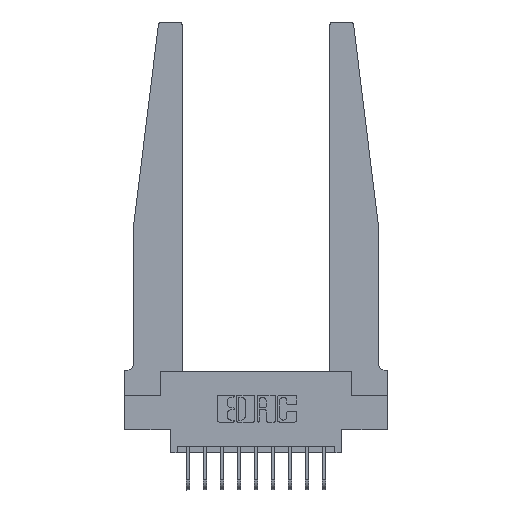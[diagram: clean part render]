
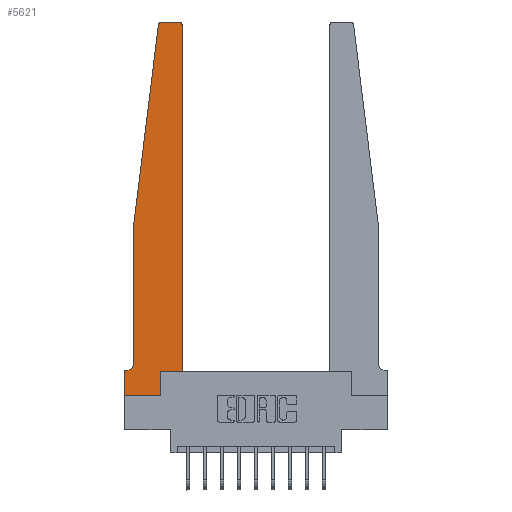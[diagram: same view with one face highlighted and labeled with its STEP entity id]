
A CAD part, top view. The second image highlights one B-rep face of the part: STEP entity #5621.
In plain terms, the highlighted planar face has unit normal (0, 0, 1).
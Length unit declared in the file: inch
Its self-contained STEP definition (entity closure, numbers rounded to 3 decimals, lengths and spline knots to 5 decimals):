
#39 = CARTESIAN_POINT ( 'NONE',  ( 0.2605, 0.18, 0.37 ) ) ;
#132 = CARTESIAN_POINT ( 'NONE',  ( 0.065, 1.25, 0.37 ) ) ;
#312 = EDGE_CURVE ( 'NONE', #11088, #11371, #10918, .T. ) ;
#405 = LINE ( 'NONE', #2624, #12284 ) ;
#443 = DIRECTION ( 'NONE',  ( 0., 0., -1. ) ) ;
#481 = CARTESIAN_POINT ( 'NONE',  ( 0.27653, 2.75, 0.37 ) ) ;
#971 = VERTEX_POINT ( 'NONE', #132 ) ;
#1061 = CARTESIAN_POINT ( 'NONE',  ( 0.2605, 0., 0.37 ) ) ;
#1147 = VECTOR ( 'NONE', #1326, 39.37008 ) ;
#1326 = DIRECTION ( 'NONE',  ( 0., -1., 0. ) ) ;
#1455 = VERTEX_POINT ( 'NONE', #39 ) ;
#1608 = CARTESIAN_POINT ( 'NONE',  ( 0., 0., 0.37 ) ) ;
#2047 = CARTESIAN_POINT ( 'NONE',  ( 0.24675, 2.72367, 0.37 ) ) ;
#2425 = CARTESIAN_POINT ( 'NONE',  ( 0., 0.1875, 0.37 ) ) ;
#2616 = AXIS2_PLACEMENT_3D ( 'NONE', #9842, #3272, #5939 ) ;
#2624 = CARTESIAN_POINT ( 'NONE',  ( 0.25, 2.75, 0.37 ) ) ;
#2648 = CARTESIAN_POINT ( 'NONE',  ( 0.065, 1.25, 0.37 ) ) ;
#2715 = CARTESIAN_POINT ( 'NONE',  ( 0., 0., 0.37 ) ) ;
#2930 = DIRECTION ( 'NONE',  ( 0., 1., 0. ) ) ;
#2935 = CARTESIAN_POINT ( 'NONE',  ( 0.425, 0.18, 0.37 ) ) ;
#3244 = DIRECTION ( 'NONE',  ( -1., 0., 0. ) ) ;
#3258 = ORIENTED_EDGE ( 'NONE', *, *, #13320, .T. ) ;
#3272 = DIRECTION ( 'NONE',  ( 0., 0., 1. ) ) ;
#3311 = EDGE_CURVE ( 'NONE', #971, #10964, #10411, .T. ) ;
#3678 = LINE ( 'NONE', #1608, #16858 ) ;
#4078 = VECTOR ( 'NONE', #11963, 39.37008 ) ;
#4135 = DIRECTION ( 'NONE',  ( 0., -1., 0. ) ) ;
#4272 = DIRECTION ( 'NONE',  ( 0., 1., 0. ) ) ;
#4403 = VERTEX_POINT ( 'NONE', #2715 ) ;
#4493 = ORIENTED_EDGE ( 'NONE', *, *, #5372, .T. ) ;
#4907 = EDGE_CURVE ( 'NONE', #15479, #6519, #12142, .T. ) ;
#4916 = ORIENTED_EDGE ( 'NONE', *, *, #8691, .T. ) ;
#4961 = CARTESIAN_POINT ( 'NONE',  ( 0.425, 0.18, 0.37 ) ) ;
#5153 = CARTESIAN_POINT ( 'NONE',  ( 0.065, 1.25, 0.37 ) ) ;
#5372 = EDGE_CURVE ( 'NONE', #13946, #4403, #3678, .T. ) ;
#5422 = CARTESIAN_POINT ( 'NONE',  ( 0.425, 0.18, 0.37 ) ) ;
#5621 = ADVANCED_FACE ( 'NONE', ( #15996 ), #6096, .T. ) ;
#5939 = DIRECTION ( 'NONE',  ( 1., 0., 0. ) ) ;
#6015 = VERTEX_POINT ( 'NONE', #16826 ) ;
#6096 = PLANE ( 'NONE',  #6764 ) ;
#6401 = DIRECTION ( 'NONE',  ( 1., 0., 0. ) ) ;
#6519 = VERTEX_POINT ( 'NONE', #12060 ) ;
#6546 = VECTOR ( 'NONE', #2930, 39.37008 ) ;
#6622 = ORIENTED_EDGE ( 'NONE', *, *, #4907, .T. ) ;
#6764 = AXIS2_PLACEMENT_3D ( 'NONE', #13968, #7461, #12772 ) ;
#6768 = EDGE_CURVE ( 'NONE', #6519, #11088, #405, .T. ) ;
#6993 = ORIENTED_EDGE ( 'NONE', *, *, #6768, .T. ) ;
#7461 = DIRECTION ( 'NONE',  ( 0., 0., 1. ) ) ;
#7664 = LINE ( 'NONE', #14934, #15677 ) ;
#7712 = CIRCLE ( 'NONE', #9263, 0.05 ) ;
#8344 = EDGE_CURVE ( 'NONE', #9085, #15479, #9742, .T. ) ;
#8691 = EDGE_CURVE ( 'NONE', #4403, #10306, #7664, .T. ) ;
#9085 = VERTEX_POINT ( 'NONE', #4961 ) ;
#9171 = LINE ( 'NONE', #9358, #6546 ) ;
#9263 = AXIS2_PLACEMENT_3D ( 'NONE', #14903, #443, #10866 ) ;
#9358 = CARTESIAN_POINT ( 'NONE',  ( 0.2605, 0.18, 0.37 ) ) ;
#9527 = LINE ( 'NONE', #5153, #10561 ) ;
#9556 = ORIENTED_EDGE ( 'NONE', *, *, #14585, .T. ) ;
#9742 = LINE ( 'NONE', #2935, #14013 ) ;
#9774 = DIRECTION ( 'NONE',  ( 1., 0., 0. ) ) ;
#9812 = ORIENTED_EDGE ( 'NONE', *, *, #11893, .T. ) ;
#9842 = CARTESIAN_POINT ( 'NONE',  ( 0.395, 2.72, 0.37 ) ) ;
#9883 = VECTOR ( 'NONE', #10895, 39.37008 ) ;
#10177 = AXIS2_PLACEMENT_3D ( 'NONE', #14450, #15793, #6401 ) ;
#10306 = VERTEX_POINT ( 'NONE', #1061 ) ;
#10411 = LINE ( 'NONE', #2648, #1147 ) ;
#10561 = VECTOR ( 'NONE', #14338, 39.37008 ) ;
#10809 = EDGE_CURVE ( 'NONE', #11371, #971, #9527, .T. ) ;
#10866 = DIRECTION ( 'NONE',  ( -1., 0., 0. ) ) ;
#10895 = DIRECTION ( 'NONE',  ( -1., 0., 0. ) ) ;
#10918 = CIRCLE ( 'NONE', #10177, 0.03 ) ;
#10964 = VERTEX_POINT ( 'NONE', #16655 ) ;
#11088 = VERTEX_POINT ( 'NONE', #481 ) ;
#11371 = VERTEX_POINT ( 'NONE', #2047 ) ;
#11667 = EDGE_CURVE ( 'NONE', #6015, #13946, #12719, .T. ) ;
#11807 = ORIENTED_EDGE ( 'NONE', *, *, #11667, .T. ) ;
#11893 = EDGE_CURVE ( 'NONE', #1455, #9085, #15828, .T. ) ;
#11963 = DIRECTION ( 'NONE',  ( 1., 0., 0. ) ) ;
#12060 = CARTESIAN_POINT ( 'NONE',  ( 0.395, 2.75, 0.37 ) ) ;
#12085 = CARTESIAN_POINT ( 'NONE',  ( 0.065, 0.1875, 0.37 ) ) ;
#12142 = CIRCLE ( 'NONE', #2616, 0.03 ) ;
#12284 = VECTOR ( 'NONE', #3244, 39.37008 ) ;
#12389 = ORIENTED_EDGE ( 'NONE', *, *, #10809, .T. ) ;
#12719 = LINE ( 'NONE', #12085, #9883 ) ;
#12772 = DIRECTION ( 'NONE',  ( 1., 0., 0. ) ) ;
#13320 = EDGE_CURVE ( 'NONE', #10964, #6015, #7712, .T. ) ;
#13843 = ORIENTED_EDGE ( 'NONE', *, *, #8344, .T. ) ;
#13946 = VERTEX_POINT ( 'NONE', #2425 ) ;
#13968 = CARTESIAN_POINT ( 'NONE',  ( 0., 0.1875, 0.37 ) ) ;
#14013 = VECTOR ( 'NONE', #4272, 39.37008 ) ;
#14338 = DIRECTION ( 'NONE',  ( -0.122, -0.992, 0. ) ) ;
#14450 = CARTESIAN_POINT ( 'NONE',  ( 0.27653, 2.72, 0.37 ) ) ;
#14585 = EDGE_CURVE ( 'NONE', #10306, #1455, #9171, .T. ) ;
#14903 = CARTESIAN_POINT ( 'NONE',  ( 0.015, 0.2375, 0.37 ) ) ;
#14934 = CARTESIAN_POINT ( 'NONE',  ( 0., 0., 0.37 ) ) ;
#15479 = VERTEX_POINT ( 'NONE', #16150 ) ;
#15608 = ORIENTED_EDGE ( 'NONE', *, *, #312, .T. ) ;
#15677 = VECTOR ( 'NONE', #9774, 39.37008 ) ;
#15793 = DIRECTION ( 'NONE',  ( 0., 0., 1. ) ) ;
#15828 = LINE ( 'NONE', #5422, #4078 ) ;
#15996 = FACE_OUTER_BOUND ( 'NONE', #16376, .T. ) ;
#16150 = CARTESIAN_POINT ( 'NONE',  ( 0.425, 2.72, 0.37 ) ) ;
#16376 = EDGE_LOOP ( 'NONE', ( #6993, #15608, #12389, #16982, #3258, #11807, #4493, #4916, #9556, #9812, #13843, #6622 ) ) ;
#16655 = CARTESIAN_POINT ( 'NONE',  ( 0.065, 0.2375, 0.37 ) ) ;
#16826 = CARTESIAN_POINT ( 'NONE',  ( 0.015, 0.1875, 0.37 ) ) ;
#16858 = VECTOR ( 'NONE', #4135, 39.37008 ) ;
#16982 = ORIENTED_EDGE ( 'NONE', *, *, #3311, .T. ) ;
